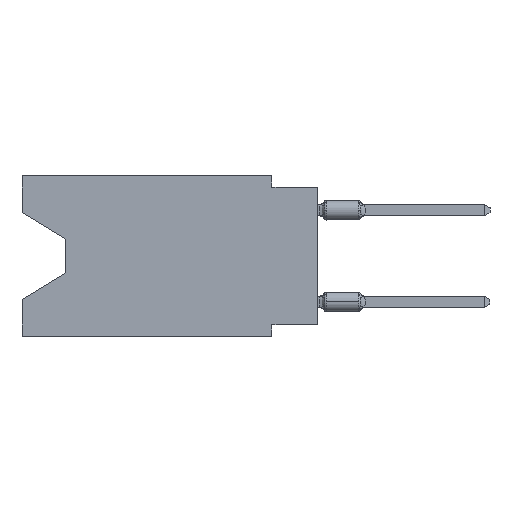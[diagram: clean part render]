
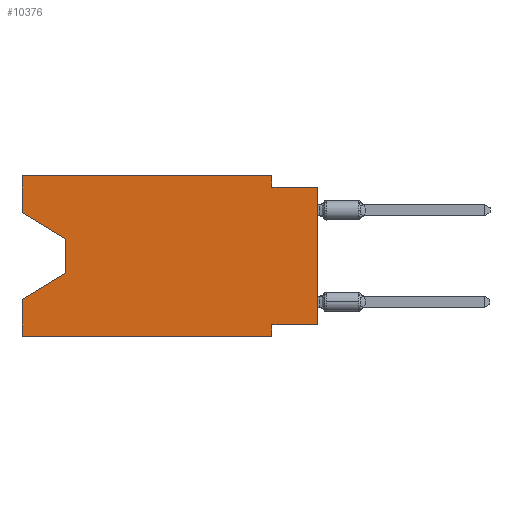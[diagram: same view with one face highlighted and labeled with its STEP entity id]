
A CAD part, left-side view. The second image highlights one B-rep face of the part: STEP entity #10376.
In plain terms, the highlighted planar face has unit normal (-1, 0, 0).
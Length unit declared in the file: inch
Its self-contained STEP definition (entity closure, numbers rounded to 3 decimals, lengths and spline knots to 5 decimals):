
#294 = CARTESIAN_POINT ( 'NONE',  ( 0., 0.55, -0.212 ) ) ;
#1061 = DIRECTION ( 'NONE',  ( 0., 0.855, -0.519 ) ) ;
#1659 = ORIENTED_EDGE ( 'NONE', *, *, #38932, .F. ) ;
#1732 = CARTESIAN_POINT ( 'NONE',  ( 0., 0., -0.325 ) ) ;
#1735 = CARTESIAN_POINT ( 'NONE',  ( 0., 0.55, -0.138 ) ) ;
#2089 = ORIENTED_EDGE ( 'NONE', *, *, #10694, .F. ) ;
#2097 = VECTOR ( 'NONE', #35981, 39.37008 ) ;
#2366 = ORIENTED_EDGE ( 'NONE', *, *, #32128, .T. ) ;
#3722 = VECTOR ( 'NONE', #36748, 39.37008 ) ;
#3798 = CARTESIAN_POINT ( 'NONE',  ( 0., 0., -0.325 ) ) ;
#4316 = ORIENTED_EDGE ( 'NONE', *, *, #20820, .F. ) ;
#4678 = CARTESIAN_POINT ( 'NONE',  ( 0., 0.55, -0.138 ) ) ;
#5160 = LINE ( 'NONE', #1732, #33113 ) ;
#5307 = PLANE ( 'NONE',  #37701 ) ;
#5637 = CARTESIAN_POINT ( 'NONE',  ( 0., 0.645, 0. ) ) ;
#7591 = LINE ( 'NONE', #4678, #34798 ) ;
#7703 = LINE ( 'NONE', #22644, #37860 ) ;
#8232 = CARTESIAN_POINT ( 'NONE',  ( 0., 0.645, 0. ) ) ;
#8382 = ORIENTED_EDGE ( 'NONE', *, *, #37127, .T. ) ;
#8960 = FACE_OUTER_BOUND ( 'NONE', #26843, .T. ) ;
#9254 = VECTOR ( 'NONE', #24729, 39.37008 ) ;
#10376 = ADVANCED_FACE ( 'NONE', ( #8960 ), #5307, .F. ) ;
#10694 = EDGE_CURVE ( 'NONE', #31974, #27637, #12099, .T. ) ;
#11629 = CARTESIAN_POINT ( 'NONE',  ( 0., 0.1, -0.35 ) ) ;
#12099 = LINE ( 'NONE', #37786, #29858 ) ;
#12531 = VERTEX_POINT ( 'NONE', #32266 ) ;
#12751 = LINE ( 'NONE', #5637, #2097 ) ;
#12960 = EDGE_CURVE ( 'NONE', #14415, #31974, #7703, .T. ) ;
#13719 = ORIENTED_EDGE ( 'NONE', *, *, #47057, .T. ) ;
#14415 = VERTEX_POINT ( 'NONE', #39792 ) ;
#15540 = EDGE_CURVE ( 'NONE', #12531, #22512, #31318, .T. ) ;
#15769 = LINE ( 'NONE', #11629, #43522 ) ;
#15798 = EDGE_CURVE ( 'NONE', #47771, #25548, #15769, .T. ) ;
#16399 = CARTESIAN_POINT ( 'NONE',  ( 0., 0.645, -0.08025 ) ) ;
#16657 = DIRECTION ( 'NONE',  ( 0., 1., 0. ) ) ;
#16841 = CARTESIAN_POINT ( 'NONE',  ( 0., 0.645, 0. ) ) ;
#17732 = EDGE_CURVE ( 'NONE', #43074, #47771, #5160, .T. ) ;
#17910 = CARTESIAN_POINT ( 'NONE',  ( 0., 0.645, 0. ) ) ;
#18080 = LINE ( 'NONE', #29085, #20425 ) ;
#18470 = DIRECTION ( 'NONE',  ( 0., 0., -1. ) ) ;
#19263 = DIRECTION ( 'NONE',  ( 0., 0., -1. ) ) ;
#19596 = DIRECTION ( 'NONE',  ( 0., -0.855, -0.519 ) ) ;
#19692 = LINE ( 'NONE', #45614, #31108 ) ;
#19941 = DIRECTION ( 'NONE',  ( 0., -1., 0. ) ) ;
#20262 = DIRECTION ( 'NONE',  ( 1., 0., 0. ) ) ;
#20425 = VECTOR ( 'NONE', #21993, 39.37008 ) ;
#20820 = EDGE_CURVE ( 'NONE', #36952, #14415, #28127, .T. ) ;
#20826 = LINE ( 'NONE', #28180, #9254 ) ;
#21819 = CARTESIAN_POINT ( 'NONE',  ( 0., 0.645, -0.35 ) ) ;
#21993 = DIRECTION ( 'NONE',  ( 0., 0., 1. ) ) ;
#22512 = VERTEX_POINT ( 'NONE', #1735 ) ;
#22644 = CARTESIAN_POINT ( 'NONE',  ( 0., 0.1, 0. ) ) ;
#22739 = EDGE_CURVE ( 'NONE', #43074, #27637, #20826, .T. ) ;
#24729 = DIRECTION ( 'NONE',  ( 0., 0., 1. ) ) ;
#25548 = VERTEX_POINT ( 'NONE', #26390 ) ;
#26390 = CARTESIAN_POINT ( 'NONE',  ( 0., 0.1, -0.35 ) ) ;
#26843 = EDGE_LOOP ( 'NONE', ( #46471, #8382, #13719, #40453, #2366, #36574, #45442, #37667, #2089, #27238, #4316, #1659 ) ) ;
#27238 = ORIENTED_EDGE ( 'NONE', *, *, #12960, .F. ) ;
#27481 = CARTESIAN_POINT ( 'NONE',  ( 0., 0.1, -0.025 ) ) ;
#27637 = VERTEX_POINT ( 'NONE', #36323 ) ;
#27953 = CARTESIAN_POINT ( 'NONE',  ( 0., 0.645, -0.26975 ) ) ;
#28127 = LINE ( 'NONE', #16841, #30222 ) ;
#28180 = CARTESIAN_POINT ( 'NONE',  ( 0., 0., 0. ) ) ;
#29085 = CARTESIAN_POINT ( 'NONE',  ( 0., 0.645, 0. ) ) ;
#29858 = VECTOR ( 'NONE', #19941, 39.37008 ) ;
#30222 = VECTOR ( 'NONE', #43047, 39.37008 ) ;
#30683 = DIRECTION ( 'NONE',  ( 0., 0., -1. ) ) ;
#31108 = VECTOR ( 'NONE', #1061, 39.37008 ) ;
#31318 = LINE ( 'NONE', #16399, #33227 ) ;
#31974 = VERTEX_POINT ( 'NONE', #27481 ) ;
#32058 = VERTEX_POINT ( 'NONE', #27953 ) ;
#32128 = EDGE_CURVE ( 'NONE', #36562, #25548, #47760, .T. ) ;
#32266 = CARTESIAN_POINT ( 'NONE',  ( 0., 0.645, -0.08025 ) ) ;
#33113 = VECTOR ( 'NONE', #16657, 39.37008 ) ;
#33227 = VECTOR ( 'NONE', #19596, 39.37008 ) ;
#34798 = VECTOR ( 'NONE', #45045, 39.37008 ) ;
#35715 = EDGE_CURVE ( 'NONE', #36562, #32058, #18080, .T. ) ;
#35981 = DIRECTION ( 'NONE',  ( 0., 0., 1. ) ) ;
#36323 = CARTESIAN_POINT ( 'NONE',  ( 0., 0., -0.025 ) ) ;
#36562 = VERTEX_POINT ( 'NONE', #48289 ) ;
#36574 = ORIENTED_EDGE ( 'NONE', *, *, #15798, .F. ) ;
#36748 = DIRECTION ( 'NONE',  ( 0., -1., 0. ) ) ;
#36952 = VERTEX_POINT ( 'NONE', #17910 ) ;
#37127 = EDGE_CURVE ( 'NONE', #22512, #48069, #7591, .T. ) ;
#37667 = ORIENTED_EDGE ( 'NONE', *, *, #22739, .T. ) ;
#37701 = AXIS2_PLACEMENT_3D ( 'NONE', #8232, #20262, #19263 ) ;
#37786 = CARTESIAN_POINT ( 'NONE',  ( 0., 0., -0.025 ) ) ;
#37812 = CARTESIAN_POINT ( 'NONE',  ( 0., 0.1, -0.325 ) ) ;
#37860 = VECTOR ( 'NONE', #18470, 39.37008 ) ;
#38932 = EDGE_CURVE ( 'NONE', #12531, #36952, #12751, .T. ) ;
#39792 = CARTESIAN_POINT ( 'NONE',  ( 0., 0.1, 0. ) ) ;
#40453 = ORIENTED_EDGE ( 'NONE', *, *, #35715, .F. ) ;
#43047 = DIRECTION ( 'NONE',  ( 0., -1., 0. ) ) ;
#43074 = VERTEX_POINT ( 'NONE', #3798 ) ;
#43522 = VECTOR ( 'NONE', #30683, 39.37008 ) ;
#45045 = DIRECTION ( 'NONE',  ( 0., 0., -1. ) ) ;
#45442 = ORIENTED_EDGE ( 'NONE', *, *, #17732, .F. ) ;
#45614 = CARTESIAN_POINT ( 'NONE',  ( 0., 0.55, -0.212 ) ) ;
#46471 = ORIENTED_EDGE ( 'NONE', *, *, #15540, .T. ) ;
#47057 = EDGE_CURVE ( 'NONE', #48069, #32058, #19692, .T. ) ;
#47760 = LINE ( 'NONE', #21819, #3722 ) ;
#47771 = VERTEX_POINT ( 'NONE', #37812 ) ;
#48069 = VERTEX_POINT ( 'NONE', #294 ) ;
#48289 = CARTESIAN_POINT ( 'NONE',  ( 0., 0.645, -0.35 ) ) ;
